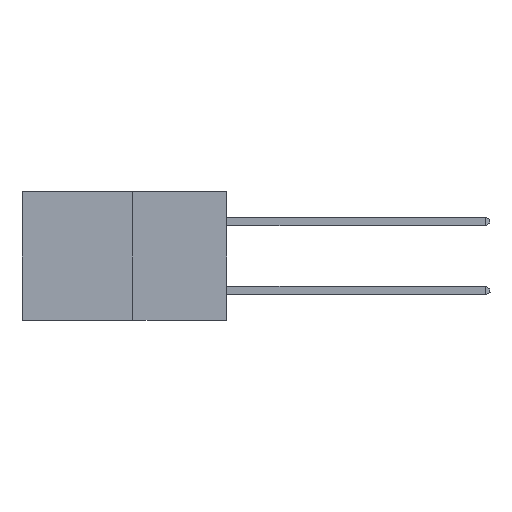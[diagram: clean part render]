
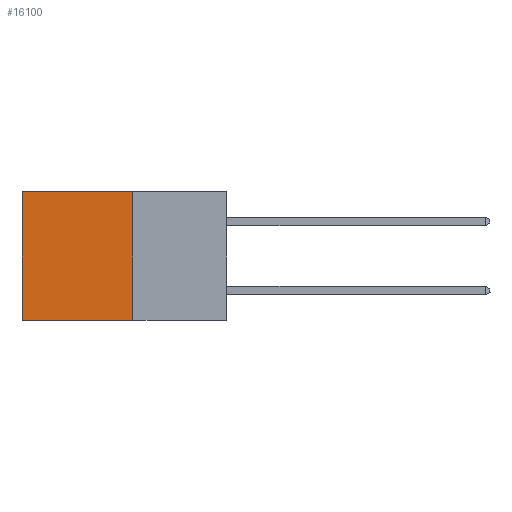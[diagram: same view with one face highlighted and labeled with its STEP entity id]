
A CAD part, left-side view. The second image highlights one B-rep face of the part: STEP entity #16100.
In plain terms, the highlighted planar face has unit normal (-1, 0, 0).
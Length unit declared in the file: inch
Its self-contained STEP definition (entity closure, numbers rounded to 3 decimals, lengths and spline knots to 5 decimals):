
#95 = CARTESIAN_POINT ( 'NONE',  ( 0.277, 0.27, -0.37 ) ) ;
#1339 = LINE ( 'NONE', #18642, #22178 ) ;
#1386 = PLANE ( 'NONE',  #4116 ) ;
#2322 = EDGE_CURVE ( 'NONE', #18446, #16007, #21779, .T. ) ;
#2825 = VECTOR ( 'NONE', #24948, 39.37008 ) ;
#3476 = DIRECTION ( 'NONE',  ( 1., 0., 0. ) ) ;
#4030 = DIRECTION ( 'NONE',  ( 0., 0., -1. ) ) ;
#4116 = AXIS2_PLACEMENT_3D ( 'NONE', #20089, #3476, #18106 ) ;
#5359 = ORIENTED_EDGE ( 'NONE', *, *, #11053, .T. ) ;
#6350 = CARTESIAN_POINT ( 'NONE',  ( 0.277, 0.59, -0.37 ) ) ;
#6585 = CARTESIAN_POINT ( 'NONE',  ( 0.277, 0.27, 0. ) ) ;
#8262 = CARTESIAN_POINT ( 'NONE',  ( 0.277, 0.27, -0.37 ) ) ;
#8761 = ORIENTED_EDGE ( 'NONE', *, *, #18654, .F. ) ;
#8887 = VERTEX_POINT ( 'NONE', #95 ) ;
#11053 = EDGE_CURVE ( 'NONE', #16007, #17315, #23269, .T. ) ;
#11509 = CARTESIAN_POINT ( 'NONE',  ( 0.277, 0.59, -0.37 ) ) ;
#15681 = FACE_OUTER_BOUND ( 'NONE', #17301, .T. ) ;
#15944 = ORIENTED_EDGE ( 'NONE', *, *, #2322, .T. ) ;
#16007 = VERTEX_POINT ( 'NONE', #26007 ) ;
#16100 = ADVANCED_FACE ( 'NONE', ( #15681 ), #1386, .F. ) ;
#16268 = EDGE_CURVE ( 'NONE', #18446, #8887, #1339, .T. ) ;
#16401 = DIRECTION ( 'NONE',  ( 0., 1., 0. ) ) ;
#17301 = EDGE_LOOP ( 'NONE', ( #5359, #8761, #21079, #15944 ) ) ;
#17315 = VERTEX_POINT ( 'NONE', #6350 ) ;
#17813 = VECTOR ( 'NONE', #23998, 39.37008 ) ;
#18106 = DIRECTION ( 'NONE',  ( 0., 0., -1. ) ) ;
#18446 = VERTEX_POINT ( 'NONE', #24330 ) ;
#18642 = CARTESIAN_POINT ( 'NONE',  ( 0.277, 0.27, -0.37 ) ) ;
#18654 = EDGE_CURVE ( 'NONE', #8887, #17315, #24953, .T. ) ;
#20089 = CARTESIAN_POINT ( 'NONE',  ( 0.277, 0.27, -0.37 ) ) ;
#21079 = ORIENTED_EDGE ( 'NONE', *, *, #16268, .F. ) ;
#21115 = VECTOR ( 'NONE', #16401, 39.37008 ) ;
#21779 = LINE ( 'NONE', #6585, #21115 ) ;
#22178 = VECTOR ( 'NONE', #4030, 39.37008 ) ;
#23269 = LINE ( 'NONE', #11509, #17813 ) ;
#23998 = DIRECTION ( 'NONE',  ( 0., 0., -1. ) ) ;
#24330 = CARTESIAN_POINT ( 'NONE',  ( 0.277, 0.27, 0. ) ) ;
#24948 = DIRECTION ( 'NONE',  ( 0., 1., 0. ) ) ;
#24953 = LINE ( 'NONE', #8262, #2825 ) ;
#26007 = CARTESIAN_POINT ( 'NONE',  ( 0.277, 0.59, 0. ) ) ;
